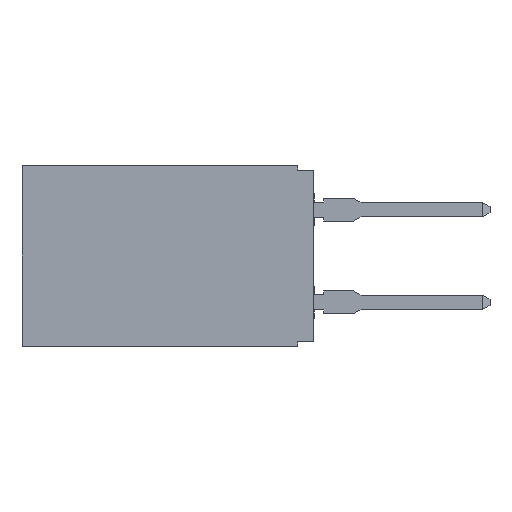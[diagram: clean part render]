
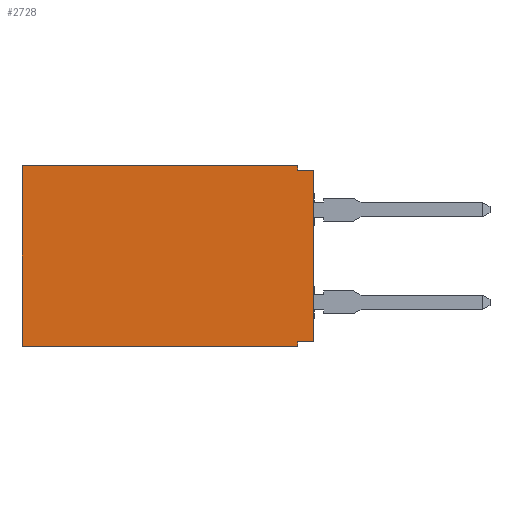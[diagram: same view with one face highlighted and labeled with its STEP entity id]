
A CAD part, left-side view. The second image highlights one B-rep face of the part: STEP entity #2728.
In plain terms, the highlighted planar face has unit normal (-1, 0, 0).
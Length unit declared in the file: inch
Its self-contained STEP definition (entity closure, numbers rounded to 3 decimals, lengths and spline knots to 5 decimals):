
#15 = VERTEX_POINT ( 'NONE', #1166 ) ;
#274 = CARTESIAN_POINT ( 'NONE',  ( -0.187, 0., 0. ) ) ;
#331 = DIRECTION ( 'NONE',  ( 0., 1., 0. ) ) ;
#332 = VERTEX_POINT ( 'NONE', #3375 ) ;
#418 = CARTESIAN_POINT ( 'NONE',  ( -0.187, 0.595, 0.195 ) ) ;
#472 = EDGE_CURVE ( 'NONE', #2531, #3768, #6027, .T. ) ;
#476 = EDGE_CURVE ( 'NONE', #737, #6578, #4954, .T. ) ;
#495 = CARTESIAN_POINT ( 'NONE',  ( -0.187, 0.595, -0.195 ) ) ;
#547 = ORIENTED_EDGE ( 'NONE', *, *, #1631, .F. ) ;
#644 = EDGE_CURVE ( 'NONE', #3061, #2531, #5732, .T. ) ;
#712 = LINE ( 'NONE', #1823, #2755 ) ;
#737 = VERTEX_POINT ( 'NONE', #3778 ) ;
#831 = EDGE_LOOP ( 'NONE', ( #2756, #2991, #2881, #4378, #2100, #2944, #4853, #547 ) ) ;
#936 = DIRECTION ( 'NONE',  ( 0., -1., 0. ) ) ;
#1166 = CARTESIAN_POINT ( 'NONE',  ( -0.187, -0.035, -0.185 ) ) ;
#1360 = DIRECTION ( 'NONE',  ( 0., 0., -1. ) ) ;
#1631 = EDGE_CURVE ( 'NONE', #332, #3061, #4901, .T. ) ;
#1641 = EDGE_CURVE ( 'NONE', #2163, #6578, #2336, .T. ) ;
#1741 = FACE_OUTER_BOUND ( 'NONE', #831, .T. ) ;
#1823 = CARTESIAN_POINT ( 'NONE',  ( -0.187, -0.035, -0.185 ) ) ;
#2100 = ORIENTED_EDGE ( 'NONE', *, *, #2710, .F. ) ;
#2144 = PLANE ( 'NONE',  #5165 ) ;
#2163 = VERTEX_POINT ( 'NONE', #3742 ) ;
#2257 = CARTESIAN_POINT ( 'NONE',  ( -0.187, 0., 0.185 ) ) ;
#2295 = CARTESIAN_POINT ( 'NONE',  ( -0.187, 0.595, 0.195 ) ) ;
#2336 = LINE ( 'NONE', #5949, #4933 ) ;
#2422 = CARTESIAN_POINT ( 'NONE',  ( -0.187, -0.035, 0.185 ) ) ;
#2491 = DIRECTION ( 'NONE',  ( 0., 0., -1. ) ) ;
#2492 = CARTESIAN_POINT ( 'NONE',  ( -0.187, 0.595, 0.195 ) ) ;
#2531 = VERTEX_POINT ( 'NONE', #4977 ) ;
#2556 = DIRECTION ( 'NONE',  ( 0., 1., 0. ) ) ;
#2628 = LINE ( 'NONE', #5146, #3187 ) ;
#2710 = EDGE_CURVE ( 'NONE', #3768, #2163, #6054, .T. ) ;
#2728 = ADVANCED_FACE ( 'NONE', ( #1741 ), #2144, .F. ) ;
#2755 = VECTOR ( 'NONE', #4354, 39.37008 ) ;
#2756 = ORIENTED_EDGE ( 'NONE', *, *, #3711, .T. ) ;
#2879 = DIRECTION ( 'NONE',  ( 0., 0., -1. ) ) ;
#2881 = ORIENTED_EDGE ( 'NONE', *, *, #476, .T. ) ;
#2944 = ORIENTED_EDGE ( 'NONE', *, *, #472, .F. ) ;
#2991 = ORIENTED_EDGE ( 'NONE', *, *, #4167, .F. ) ;
#3061 = VERTEX_POINT ( 'NONE', #6010 ) ;
#3187 = VECTOR ( 'NONE', #2491, 39.37008 ) ;
#3323 = VECTOR ( 'NONE', #1360, 39.37008 ) ;
#3375 = CARTESIAN_POINT ( 'NONE',  ( -0.187, 0., -0.185 ) ) ;
#3683 = VECTOR ( 'NONE', #4542, 39.37008 ) ;
#3690 = VECTOR ( 'NONE', #2556, 39.37008 ) ;
#3711 = EDGE_CURVE ( 'NONE', #332, #15, #712, .T. ) ;
#3742 = CARTESIAN_POINT ( 'NONE',  ( -0.187, 0., 0.195 ) ) ;
#3768 = VERTEX_POINT ( 'NONE', #2295 ) ;
#3778 = CARTESIAN_POINT ( 'NONE',  ( -0.187, -0.035, 0.185 ) ) ;
#4167 = EDGE_CURVE ( 'NONE', #737, #15, #2628, .T. ) ;
#4168 = DIRECTION ( 'NONE',  ( 1., 0., 0. ) ) ;
#4354 = DIRECTION ( 'NONE',  ( 0., -1., 0. ) ) ;
#4378 = ORIENTED_EDGE ( 'NONE', *, *, #1641, .F. ) ;
#4542 = DIRECTION ( 'NONE',  ( 0., 0., 1. ) ) ;
#4624 = VECTOR ( 'NONE', #936, 39.37008 ) ;
#4771 = CARTESIAN_POINT ( 'NONE',  ( -0.187, 0.595, 0.195 ) ) ;
#4853 = ORIENTED_EDGE ( 'NONE', *, *, #644, .F. ) ;
#4901 = LINE ( 'NONE', #274, #3323 ) ;
#4933 = VECTOR ( 'NONE', #2879, 39.37008 ) ;
#4954 = LINE ( 'NONE', #2422, #5177 ) ;
#4977 = CARTESIAN_POINT ( 'NONE',  ( -0.187, 0.595, -0.195 ) ) ;
#5146 = CARTESIAN_POINT ( 'NONE',  ( -0.187, -0.035, 0.195 ) ) ;
#5165 = AXIS2_PLACEMENT_3D ( 'NONE', #4771, #4168, #5821 ) ;
#5177 = VECTOR ( 'NONE', #331, 39.37008 ) ;
#5732 = LINE ( 'NONE', #495, #3690 ) ;
#5821 = DIRECTION ( 'NONE',  ( 0., 0., -1. ) ) ;
#5949 = CARTESIAN_POINT ( 'NONE',  ( -0.187, 0., 0. ) ) ;
#6010 = CARTESIAN_POINT ( 'NONE',  ( -0.187, 0., -0.195 ) ) ;
#6027 = LINE ( 'NONE', #2492, #3683 ) ;
#6054 = LINE ( 'NONE', #418, #4624 ) ;
#6578 = VERTEX_POINT ( 'NONE', #2257 ) ;
